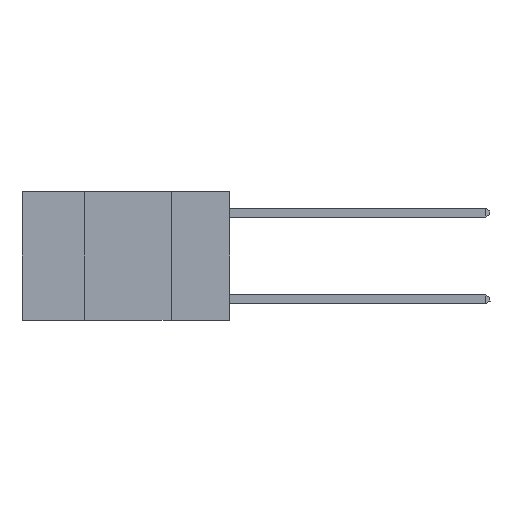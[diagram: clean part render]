
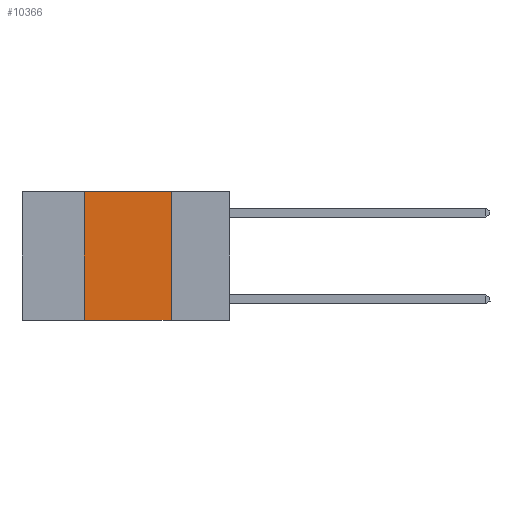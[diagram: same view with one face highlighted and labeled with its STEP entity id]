
A CAD part, left-side view. The second image highlights one B-rep face of the part: STEP entity #10366.
In plain terms, the highlighted planar face has unit normal (-1, 0, 0).
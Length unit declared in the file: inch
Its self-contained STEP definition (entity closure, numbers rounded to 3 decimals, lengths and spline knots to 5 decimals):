
#983 = CARTESIAN_POINT ( 'NONE',  ( 0., 0.17, 0. ) ) ;
#1608 = CARTESIAN_POINT ( 'NONE',  ( 0., 0.6, 0. ) ) ;
#3314 = EDGE_CURVE ( 'NONE', #17610, #13868, #13559, .T. ) ;
#4364 = EDGE_CURVE ( 'NONE', #14116, #8046, #5883, .T. ) ;
#5883 = LINE ( 'NONE', #13180, #16476 ) ;
#5898 = PLANE ( 'NONE',  #9065 ) ;
#6445 = CARTESIAN_POINT ( 'NONE',  ( 0., 0.6, -0.37 ) ) ;
#7517 = ORIENTED_EDGE ( 'NONE', *, *, #3314, .F. ) ;
#8028 = DIRECTION ( 'NONE',  ( 1., 0., 0. ) ) ;
#8046 = VERTEX_POINT ( 'NONE', #19870 ) ;
#8438 = CARTESIAN_POINT ( 'NONE',  ( 0., 0.17, -0.37 ) ) ;
#8565 = DIRECTION ( 'NONE',  ( 0., -1., 0. ) ) ;
#8921 = DIRECTION ( 'NONE',  ( 0., 0., 1. ) ) ;
#9065 = AXIS2_PLACEMENT_3D ( 'NONE', #1608, #8028, #22648 ) ;
#10241 = FACE_OUTER_BOUND ( 'NONE', #14361, .T. ) ;
#10366 = ADVANCED_FACE ( 'NONE', ( #10241 ), #5898, .F. ) ;
#11593 = CARTESIAN_POINT ( 'NONE',  ( 0., 0.6, 0. ) ) ;
#12512 = EDGE_CURVE ( 'NONE', #14116, #13868, #25003, .T. ) ;
#13180 = CARTESIAN_POINT ( 'NONE',  ( 0., 0.42, 0. ) ) ;
#13405 = VECTOR ( 'NONE', #8565, 39.37008 ) ;
#13559 = LINE ( 'NONE', #23379, #23922 ) ;
#13868 = VERTEX_POINT ( 'NONE', #8438 ) ;
#14116 = VERTEX_POINT ( 'NONE', #21615 ) ;
#14361 = EDGE_LOOP ( 'NONE', ( #7517, #20006, #15139, #21291 ) ) ;
#15139 = ORIENTED_EDGE ( 'NONE', *, *, #4364, .F. ) ;
#16476 = VECTOR ( 'NONE', #8921, 39.37008 ) ;
#17610 = VERTEX_POINT ( 'NONE', #983 ) ;
#19485 = LINE ( 'NONE', #11593, #24267 ) ;
#19870 = CARTESIAN_POINT ( 'NONE',  ( 0., 0.42, 0. ) ) ;
#20006 = ORIENTED_EDGE ( 'NONE', *, *, #24625, .F. ) ;
#21291 = ORIENTED_EDGE ( 'NONE', *, *, #12512, .T. ) ;
#21336 = DIRECTION ( 'NONE',  ( 0., 0., -1. ) ) ;
#21615 = CARTESIAN_POINT ( 'NONE',  ( 0., 0.42, -0.37 ) ) ;
#22648 = DIRECTION ( 'NONE',  ( 0., 0., -1. ) ) ;
#23379 = CARTESIAN_POINT ( 'NONE',  ( 0., 0.17, 0. ) ) ;
#23922 = VECTOR ( 'NONE', #21336, 39.37008 ) ;
#24267 = VECTOR ( 'NONE', #26145, 39.37008 ) ;
#24625 = EDGE_CURVE ( 'NONE', #8046, #17610, #19485, .T. ) ;
#25003 = LINE ( 'NONE', #6445, #13405 ) ;
#26145 = DIRECTION ( 'NONE',  ( 0., -1., 0. ) ) ;
